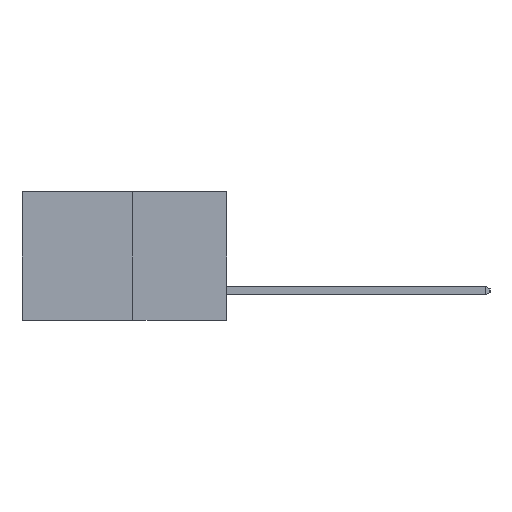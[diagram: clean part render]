
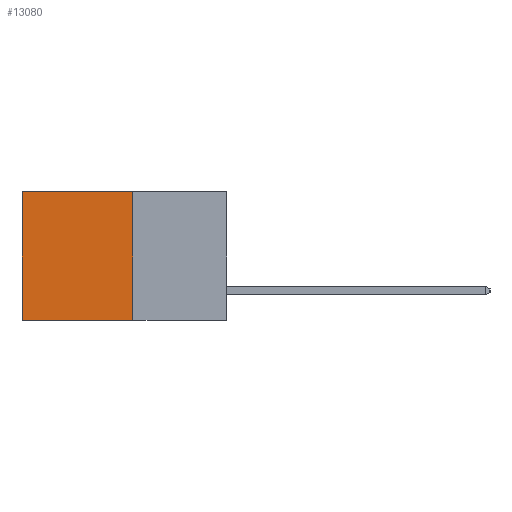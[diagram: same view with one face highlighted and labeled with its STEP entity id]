
A CAD part, left-side view. The second image highlights one B-rep face of the part: STEP entity #13080.
In plain terms, the highlighted planar face has unit normal (-1, 0, 0).
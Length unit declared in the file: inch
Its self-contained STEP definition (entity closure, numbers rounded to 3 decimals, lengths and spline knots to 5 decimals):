
#94 = CARTESIAN_POINT ( 'NONE',  ( 0.277, 0.27, 0. ) ) ;
#238 = VERTEX_POINT ( 'NONE', #8476 ) ;
#749 = CARTESIAN_POINT ( 'NONE',  ( 0.277, 0.59, -0.37 ) ) ;
#752 = DIRECTION ( 'NONE',  ( 0., 0., -1. ) ) ;
#3683 = VECTOR ( 'NONE', #13668, 39.37008 ) ;
#3746 = VECTOR ( 'NONE', #7337, 39.37008 ) ;
#3823 = ORIENTED_EDGE ( 'NONE', *, *, #10077, .T. ) ;
#3986 = LINE ( 'NONE', #11740, #6892 ) ;
#4051 = DIRECTION ( 'NONE',  ( 0., 1., 0. ) ) ;
#4335 = VERTEX_POINT ( 'NONE', #13133 ) ;
#4852 = ORIENTED_EDGE ( 'NONE', *, *, #7418, .F. ) ;
#5151 = VECTOR ( 'NONE', #11615, 39.37008 ) ;
#5552 = VERTEX_POINT ( 'NONE', #12048 ) ;
#5793 = ORIENTED_EDGE ( 'NONE', *, *, #12895, .F. ) ;
#6011 = EDGE_CURVE ( 'NONE', #7652, #238, #3986, .T. ) ;
#6104 = CARTESIAN_POINT ( 'NONE',  ( 0.277, 0.27, -0.37 ) ) ;
#6207 = EDGE_LOOP ( 'NONE', ( #3823, #4852, #5793, #10249 ) ) ;
#6242 = CARTESIAN_POINT ( 'NONE',  ( 0.277, 0.27, -0.37 ) ) ;
#6892 = VECTOR ( 'NONE', #4051, 39.37008 ) ;
#7337 = DIRECTION ( 'NONE',  ( 0., 0., -1. ) ) ;
#7341 = DIRECTION ( 'NONE',  ( 1., 0., 0. ) ) ;
#7418 = EDGE_CURVE ( 'NONE', #5552, #4335, #14226, .T. ) ;
#7652 = VERTEX_POINT ( 'NONE', #94 ) ;
#8476 = CARTESIAN_POINT ( 'NONE',  ( 0.277, 0.59, 0. ) ) ;
#9285 = CARTESIAN_POINT ( 'NONE',  ( 0.277, 0.27, -0.37 ) ) ;
#9586 = AXIS2_PLACEMENT_3D ( 'NONE', #6242, #7341, #752 ) ;
#9921 = LINE ( 'NONE', #9285, #3683 ) ;
#10077 = EDGE_CURVE ( 'NONE', #238, #4335, #12553, .T. ) ;
#10091 = FACE_OUTER_BOUND ( 'NONE', #6207, .T. ) ;
#10249 = ORIENTED_EDGE ( 'NONE', *, *, #6011, .T. ) ;
#11615 = DIRECTION ( 'NONE',  ( 0., 1., 0. ) ) ;
#11740 = CARTESIAN_POINT ( 'NONE',  ( 0.277, 0.27, 0. ) ) ;
#12048 = CARTESIAN_POINT ( 'NONE',  ( 0.277, 0.27, -0.37 ) ) ;
#12553 = LINE ( 'NONE', #749, #3746 ) ;
#12862 = PLANE ( 'NONE',  #9586 ) ;
#12895 = EDGE_CURVE ( 'NONE', #7652, #5552, #9921, .T. ) ;
#13080 = ADVANCED_FACE ( 'NONE', ( #10091 ), #12862, .F. ) ;
#13133 = CARTESIAN_POINT ( 'NONE',  ( 0.277, 0.59, -0.37 ) ) ;
#13668 = DIRECTION ( 'NONE',  ( 0., 0., -1. ) ) ;
#14226 = LINE ( 'NONE', #6104, #5151 ) ;
